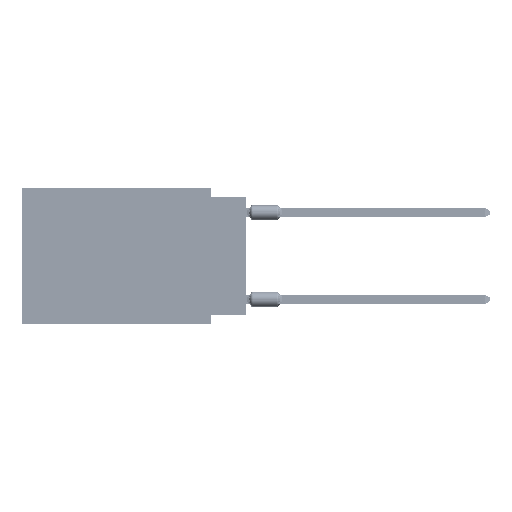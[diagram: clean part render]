
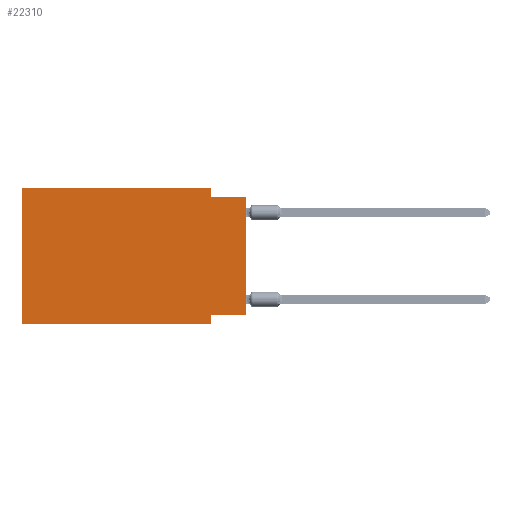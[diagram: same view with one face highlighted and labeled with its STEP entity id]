
A CAD part, left-side view. The second image highlights one B-rep face of the part: STEP entity #22310.
In plain terms, the highlighted planar face has unit normal (-1, 0, 0).
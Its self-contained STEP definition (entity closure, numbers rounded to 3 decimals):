
#271 = VECTOR ( 'NONE', #65660, 1000. ) ;
#1676 = LINE ( 'NONE', #23427, #58392 ) ;
#1884 = CARTESIAN_POINT ( 'NONE',  ( 0., 16.383, -9.906 ) ) ;
#6377 = EDGE_CURVE ( 'NONE', #64671, #16385, #61955, .T. ) ;
#7142 = VERTEX_POINT ( 'NONE', #43571 ) ;
#9002 = EDGE_CURVE ( 'NONE', #23096, #19229, #56590, .T. ) ;
#10119 = CARTESIAN_POINT ( 'NONE',  ( 0., 2.54, -9.271 ) ) ;
#12640 = LINE ( 'NONE', #45430, #35559 ) ;
#12776 = VECTOR ( 'NONE', #66946, 1000. ) ;
#12836 = EDGE_LOOP ( 'NONE', ( #39108, #26979, #60624, #69527, #64971, #49549, #24119, #53344 ) ) ;
#13216 = LINE ( 'NONE', #35636, #45731 ) ;
#14130 = DIRECTION ( 'NONE',  ( 1., 0., 0. ) ) ;
#16385 = VERTEX_POINT ( 'NONE', #37164 ) ;
#18407 = LINE ( 'NONE', #29789, #43254 ) ;
#18493 = DIRECTION ( 'NONE',  ( 0., 1., 0. ) ) ;
#19229 = VERTEX_POINT ( 'NONE', #10119 ) ;
#19484 = CARTESIAN_POINT ( 'NONE',  ( 0., 16.383, 0. ) ) ;
#22310 = ADVANCED_FACE ( 'NONE', ( #57578 ), #68273, .F. ) ;
#22938 = CARTESIAN_POINT ( 'NONE',  ( 0., 2.54, -0.635 ) ) ;
#23096 = VERTEX_POINT ( 'NONE', #62062 ) ;
#23427 = CARTESIAN_POINT ( 'NONE',  ( 0., 2.54, 0. ) ) ;
#23512 = CARTESIAN_POINT ( 'NONE',  ( 0., 0., -0.635 ) ) ;
#23630 = LINE ( 'NONE', #1884, #271 ) ;
#24119 = ORIENTED_EDGE ( 'NONE', *, *, #55163, .F. ) ;
#24796 = DIRECTION ( 'NONE',  ( 0., 0., 1. ) ) ;
#25584 = LINE ( 'NONE', #67961, #53397 ) ;
#25731 = EDGE_CURVE ( 'NONE', #7142, #31114, #25584, .T. ) ;
#26979 = ORIENTED_EDGE ( 'NONE', *, *, #6377, .F. ) ;
#29789 = CARTESIAN_POINT ( 'NONE',  ( 0., 16.383, 0. ) ) ;
#29947 = DIRECTION ( 'NONE',  ( 0., 0., -1. ) ) ;
#31114 = VERTEX_POINT ( 'NONE', #60627 ) ;
#35559 = VECTOR ( 'NONE', #49721, 1000. ) ;
#35636 = CARTESIAN_POINT ( 'NONE',  ( 0., 2.54, -9.906 ) ) ;
#36590 = EDGE_CURVE ( 'NONE', #52869, #41402, #23630, .T. ) ;
#37164 = CARTESIAN_POINT ( 'NONE',  ( 0., 0., -0.635 ) ) ;
#39108 = ORIENTED_EDGE ( 'NONE', *, *, #57187, .T. ) ;
#41402 = VERTEX_POINT ( 'NONE', #48493 ) ;
#43254 = VECTOR ( 'NONE', #24796, 1000. ) ;
#43571 = CARTESIAN_POINT ( 'NONE',  ( 0., 16.383, 0. ) ) ;
#44455 = EDGE_CURVE ( 'NONE', #31114, #64671, #1676, .T. ) ;
#45154 = DIRECTION ( 'NONE',  ( 0., 0., -1. ) ) ;
#45222 = CARTESIAN_POINT ( 'NONE',  ( 0., 0., -9.271 ) ) ;
#45430 = CARTESIAN_POINT ( 'NONE',  ( 0., 0., 0. ) ) ;
#45731 = VECTOR ( 'NONE', #29947, 1000. ) ;
#46244 = AXIS2_PLACEMENT_3D ( 'NONE', #19484, #14130, #50513 ) ;
#48493 = CARTESIAN_POINT ( 'NONE',  ( 0., 2.54, -9.906 ) ) ;
#49549 = ORIENTED_EDGE ( 'NONE', *, *, #36590, .T. ) ;
#49721 = DIRECTION ( 'NONE',  ( 0., 0., 1. ) ) ;
#50513 = DIRECTION ( 'NONE',  ( 0., 0., -1. ) ) ;
#52217 = CARTESIAN_POINT ( 'NONE',  ( 0., 16.383, -9.906 ) ) ;
#52869 = VERTEX_POINT ( 'NONE', #52217 ) ;
#52889 = EDGE_CURVE ( 'NONE', #52869, #7142, #18407, .T. ) ;
#53344 = ORIENTED_EDGE ( 'NONE', *, *, #9002, .F. ) ;
#53397 = VECTOR ( 'NONE', #53937, 1000. ) ;
#53937 = DIRECTION ( 'NONE',  ( 0., -1., 0. ) ) ;
#55163 = EDGE_CURVE ( 'NONE', #19229, #41402, #13216, .T. ) ;
#56106 = VECTOR ( 'NONE', #18493, 1000. ) ;
#56590 = LINE ( 'NONE', #45222, #56106 ) ;
#57187 = EDGE_CURVE ( 'NONE', #23096, #16385, #12640, .T. ) ;
#57578 = FACE_OUTER_BOUND ( 'NONE', #12836, .T. ) ;
#58392 = VECTOR ( 'NONE', #45154, 1000. ) ;
#60624 = ORIENTED_EDGE ( 'NONE', *, *, #44455, .F. ) ;
#60627 = CARTESIAN_POINT ( 'NONE',  ( 0., 2.54, 0. ) ) ;
#61955 = LINE ( 'NONE', #23512, #12776 ) ;
#62062 = CARTESIAN_POINT ( 'NONE',  ( 0., 0., -9.271 ) ) ;
#64671 = VERTEX_POINT ( 'NONE', #22938 ) ;
#64971 = ORIENTED_EDGE ( 'NONE', *, *, #52889, .F. ) ;
#65660 = DIRECTION ( 'NONE',  ( 0., -1., 0. ) ) ;
#66946 = DIRECTION ( 'NONE',  ( 0., -1., 0. ) ) ;
#67961 = CARTESIAN_POINT ( 'NONE',  ( 0., 16.383, 0. ) ) ;
#68273 = PLANE ( 'NONE',  #46244 ) ;
#69527 = ORIENTED_EDGE ( 'NONE', *, *, #25731, .F. ) ;
